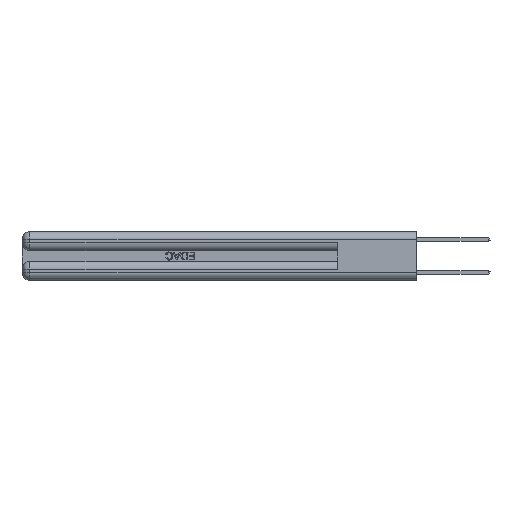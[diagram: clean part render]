
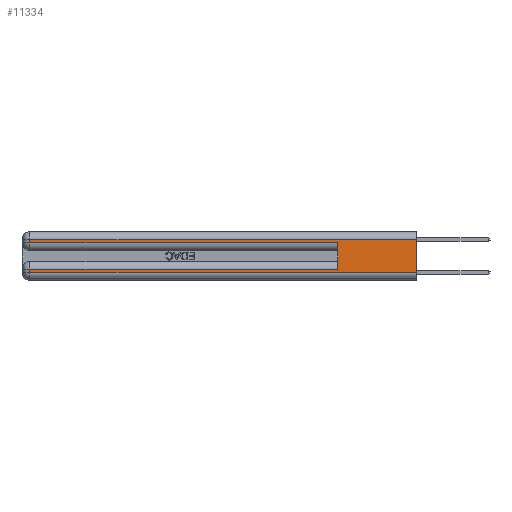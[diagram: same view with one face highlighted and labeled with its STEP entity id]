
A CAD part, left-side view. The second image highlights one B-rep face of the part: STEP entity #11334.
In plain terms, the highlighted planar face has unit normal (-1, 0, 0).
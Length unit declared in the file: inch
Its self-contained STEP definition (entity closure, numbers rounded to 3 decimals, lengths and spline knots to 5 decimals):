
#676 = ORIENTED_EDGE ( 'NONE', *, *, #22095, .F. ) ;
#1838 = DIRECTION ( 'NONE',  ( 0., 1., 0. ) ) ;
#2124 = CARTESIAN_POINT ( 'NONE',  ( 0., 0., 0.06 ) ) ;
#2385 = CARTESIAN_POINT ( 'NONE',  ( 0., 2.94, 0.285 ) ) ;
#3622 = VERTEX_POINT ( 'NONE', #2385 ) ;
#4429 = VERTEX_POINT ( 'NONE', #26389 ) ;
#4684 = ORIENTED_EDGE ( 'NONE', *, *, #24599, .T. ) ;
#4870 = CARTESIAN_POINT ( 'NONE',  ( 0., 2.94, 0.06 ) ) ;
#5026 = LINE ( 'NONE', #22850, #6086 ) ;
#5040 = CARTESIAN_POINT ( 'NONE',  ( 0., 0., 0.285 ) ) ;
#5183 = EDGE_CURVE ( 'NONE', #6314, #22500, #6582, .T. ) ;
#5487 = CARTESIAN_POINT ( 'NONE',  ( 0., 0., 0.37 ) ) ;
#5862 = CARTESIAN_POINT ( 'NONE',  ( 0., 0.6, 0.285 ) ) ;
#6086 = VECTOR ( 'NONE', #14274, 39.37008 ) ;
#6314 = VERTEX_POINT ( 'NONE', #25143 ) ;
#6460 = CARTESIAN_POINT ( 'NONE',  ( 0., 2.94, 0.37 ) ) ;
#6582 = LINE ( 'NONE', #29970, #15886 ) ;
#6819 = CARTESIAN_POINT ( 'NONE',  ( 0., 2.94, 0.37 ) ) ;
#7136 = CARTESIAN_POINT ( 'NONE',  ( 0., 2.94, 0.085 ) ) ;
#7277 = VECTOR ( 'NONE', #32049, 39.37008 ) ;
#8965 = ORIENTED_EDGE ( 'NONE', *, *, #5183, .T. ) ;
#10989 = DIRECTION ( 'NONE',  ( 0., 0., -1. ) ) ;
#11215 = VERTEX_POINT ( 'NONE', #11250 ) ;
#11250 = CARTESIAN_POINT ( 'NONE',  ( 0., 0., 0.31 ) ) ;
#11334 = ADVANCED_FACE ( 'NONE', ( #29592 ), #11905, .F. ) ;
#11905 = PLANE ( 'NONE',  #30788 ) ;
#14274 = DIRECTION ( 'NONE',  ( 0., 1., 0. ) ) ;
#15239 = DIRECTION ( 'NONE',  ( 0., -1., 0. ) ) ;
#15605 = ORIENTED_EDGE ( 'NONE', *, *, #25926, .F. ) ;
#15699 = DIRECTION ( 'NONE',  ( 0., 0., -1. ) ) ;
#15886 = VECTOR ( 'NONE', #1838, 39.37008 ) ;
#16553 = VECTOR ( 'NONE', #15239, 39.37008 ) ;
#16850 = LINE ( 'NONE', #6819, #24606 ) ;
#17188 = LINE ( 'NONE', #21668, #7277 ) ;
#18059 = VERTEX_POINT ( 'NONE', #2124 ) ;
#19002 = DIRECTION ( 'NONE',  ( 0., 0., -1. ) ) ;
#19431 = ORIENTED_EDGE ( 'NONE', *, *, #32342, .T. ) ;
#20375 = EDGE_LOOP ( 'NONE', ( #676, #22921, #19431, #31234, #15605, #8965, #4684, #22994 ) ) ;
#20907 = EDGE_CURVE ( 'NONE', #29556, #18059, #27105, .T. ) ;
#21510 = EDGE_CURVE ( 'NONE', #3622, #22948, #25205, .T. ) ;
#21668 = CARTESIAN_POINT ( 'NONE',  ( 0., 0.6, 0.145 ) ) ;
#22095 = EDGE_CURVE ( 'NONE', #11215, #18059, #26500, .T. ) ;
#22254 = CARTESIAN_POINT ( 'NONE',  ( 0., 0., 0.06 ) ) ;
#22364 = CARTESIAN_POINT ( 'NONE',  ( 0., 0., 0.37 ) ) ;
#22500 = VERTEX_POINT ( 'NONE', #7136 ) ;
#22850 = CARTESIAN_POINT ( 'NONE',  ( 0., 0., 0.31 ) ) ;
#22921 = ORIENTED_EDGE ( 'NONE', *, *, #29630, .T. ) ;
#22948 = VERTEX_POINT ( 'NONE', #5862 ) ;
#22994 = ORIENTED_EDGE ( 'NONE', *, *, #20907, .T. ) ;
#24263 = VECTOR ( 'NONE', #10989, 39.37008 ) ;
#24382 = DIRECTION ( 'NONE',  ( 0., 0., -1. ) ) ;
#24599 = EDGE_CURVE ( 'NONE', #22500, #29556, #28996, .T. ) ;
#24606 = VECTOR ( 'NONE', #19002, 39.37008 ) ;
#24703 = DIRECTION ( 'NONE',  ( 1., 0., 0. ) ) ;
#25143 = CARTESIAN_POINT ( 'NONE',  ( 0., 0.6, 0.085 ) ) ;
#25205 = LINE ( 'NONE', #5040, #16553 ) ;
#25521 = VECTOR ( 'NONE', #29808, 39.37008 ) ;
#25926 = EDGE_CURVE ( 'NONE', #6314, #22948, #17188, .T. ) ;
#26389 = CARTESIAN_POINT ( 'NONE',  ( 0., 2.94, 0.31 ) ) ;
#26500 = LINE ( 'NONE', #5487, #30453 ) ;
#27105 = LINE ( 'NONE', #22254, #25521 ) ;
#28996 = LINE ( 'NONE', #6460, #24263 ) ;
#29556 = VERTEX_POINT ( 'NONE', #4870 ) ;
#29592 = FACE_OUTER_BOUND ( 'NONE', #20375, .T. ) ;
#29630 = EDGE_CURVE ( 'NONE', #11215, #4429, #5026, .T. ) ;
#29808 = DIRECTION ( 'NONE',  ( 0., -1., 0. ) ) ;
#29970 = CARTESIAN_POINT ( 'NONE',  ( 0., 0., 0.085 ) ) ;
#30453 = VECTOR ( 'NONE', #15699, 39.37008 ) ;
#30788 = AXIS2_PLACEMENT_3D ( 'NONE', #22364, #24703, #24382 ) ;
#31234 = ORIENTED_EDGE ( 'NONE', *, *, #21510, .T. ) ;
#32049 = DIRECTION ( 'NONE',  ( 0., 0., 1. ) ) ;
#32342 = EDGE_CURVE ( 'NONE', #4429, #3622, #16850, .T. ) ;
